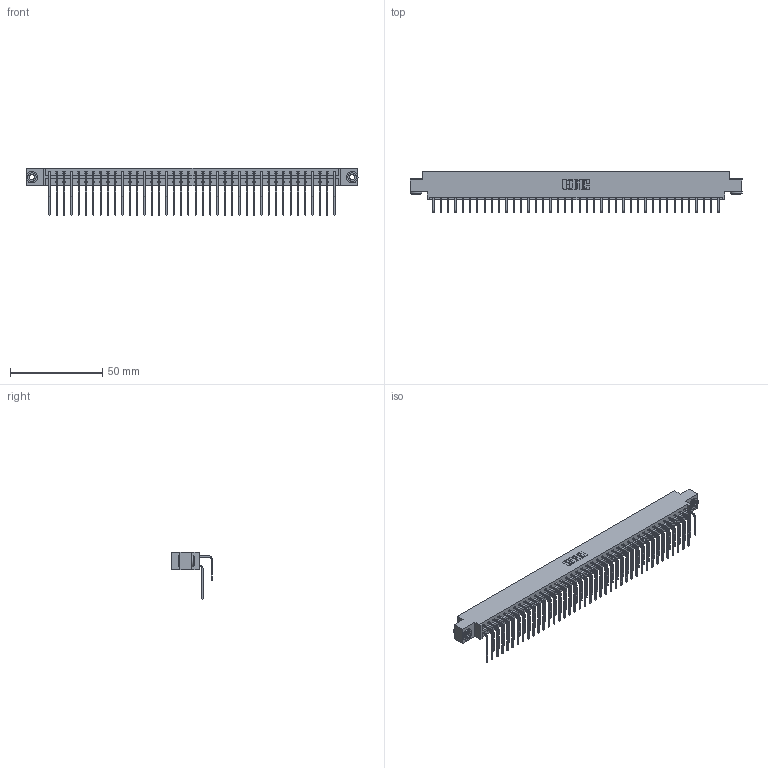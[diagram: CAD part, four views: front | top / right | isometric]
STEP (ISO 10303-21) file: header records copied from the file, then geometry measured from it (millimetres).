
FILE_DESCRIPTION (( 'STEP AP203' ), '1' );
FILE_NAME ('333-080-558-803.STEP', '2018-08-05T02:11:55', ( '' ), ( '' ), 'SwSTEP 2.0', 'SolidWorks 2016', '' );
FILE_SCHEMA (( 'CONFIG_CONTROL_DESIGN' ));
Length unit declared in the file: inch
Products named in the file (5): 333-080-558-803; 333 Part_Offset - .156 Dia - TH; 345-292-001_558 559 Tail - 1; 345-292-001_558 Tail - 2; 345-250-002_345-250-002-102
Assembly tree (83 placements, depth 2):
  333-080-558-803
    333 Part_Offset - .156 Dia - TH
    345-292-001_558 559 Tail - 1  x40
    345-292-001_558 Tail - 2  x40
    345-250-002_345-250-002-102  x2
Bounding box: 180.04 x 22.17 x 25.53 mm (x, y, z)
Volume: 18615 mm3; surface area: 24726.5 mm2
Topology: 83 solids, 83 shells, 4476 faces, 13279 edges, 8742 vertices
Faces by surface type: plane 3124, cylinder 1344, cone 8
Entity records: 28558 total; most frequent: CARTESIAN_POINT 4764, ORIENTED_EDGE 4642, DIRECTION 4087, EDGE_CURVE 2321, LINE 2129, VECTOR 2129, VERTEX_POINT 1542, AXIS2_PLACEMENT_3D 979
